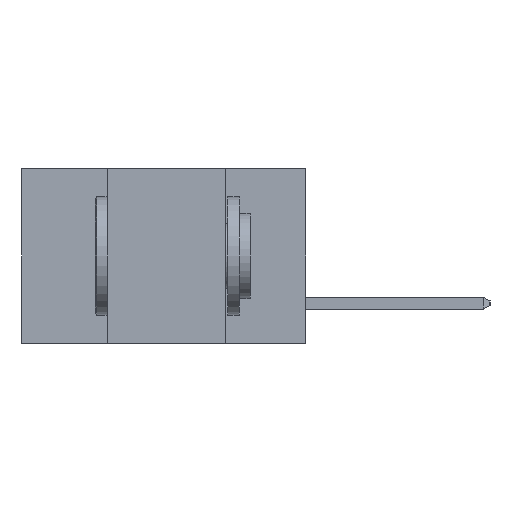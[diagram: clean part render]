
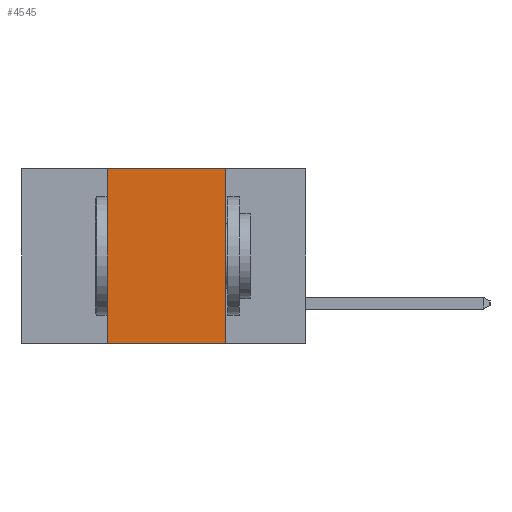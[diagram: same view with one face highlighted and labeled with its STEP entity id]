
A CAD part, left-side view. The second image highlights one B-rep face of the part: STEP entity #4545.
In plain terms, the highlighted planar face has unit normal (-1, 0, 0).
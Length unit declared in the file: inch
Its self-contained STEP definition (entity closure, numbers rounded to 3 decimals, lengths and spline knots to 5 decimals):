
#426 = LINE ( 'NONE', #20984, #14366 ) ;
#1055 = DIRECTION ( 'NONE',  ( 0., 0., 1. ) ) ;
#1083 = CARTESIAN_POINT ( 'NONE',  ( 0., 0.42, -0.37 ) ) ;
#1262 = EDGE_CURVE ( 'NONE', #13277, #11689, #426, .T. ) ;
#2244 = FACE_OUTER_BOUND ( 'NONE', #10930, .T. ) ;
#2871 = DIRECTION ( 'NONE',  ( 0., 0., -1. ) ) ;
#3153 = ORIENTED_EDGE ( 'NONE', *, *, #7551, .F. ) ;
#3324 = CARTESIAN_POINT ( 'NONE',  ( 0., 0.17, -0.37 ) ) ;
#3394 = LINE ( 'NONE', #14485, #21994 ) ;
#4510 = EDGE_CURVE ( 'NONE', #10075, #11689, #12654, .T. ) ;
#4545 = ADVANCED_FACE ( 'NONE', ( #2244 ), #21687, .F. ) ;
#5328 = ORIENTED_EDGE ( 'NONE', *, *, #4510, .F. ) ;
#5623 = CARTESIAN_POINT ( 'NONE',  ( 0., 0.17, 0. ) ) ;
#7551 = EDGE_CURVE ( 'NONE', #13277, #8636, #20561, .T. ) ;
#8636 = VERTEX_POINT ( 'NONE', #11726 ) ;
#8862 = ORIENTED_EDGE ( 'NONE', *, *, #17502, .F. ) ;
#10075 = VERTEX_POINT ( 'NONE', #5623 ) ;
#10930 = EDGE_LOOP ( 'NONE', ( #5328, #8862, #3153, #20760 ) ) ;
#11680 = VECTOR ( 'NONE', #1055, 39.37008 ) ;
#11689 = VERTEX_POINT ( 'NONE', #12304 ) ;
#11726 = CARTESIAN_POINT ( 'NONE',  ( 0., 0.42, 0. ) ) ;
#12304 = CARTESIAN_POINT ( 'NONE',  ( 0., 0.17, -0.37 ) ) ;
#12654 = LINE ( 'NONE', #3324, #16607 ) ;
#12837 = DIRECTION ( 'NONE',  ( 0., -1., 0. ) ) ;
#13277 = VERTEX_POINT ( 'NONE', #13948 ) ;
#13948 = CARTESIAN_POINT ( 'NONE',  ( 0., 0.42, -0.37 ) ) ;
#14366 = VECTOR ( 'NONE', #21563, 39.37008 ) ;
#14485 = CARTESIAN_POINT ( 'NONE',  ( 0., 0.6, 0. ) ) ;
#15072 = AXIS2_PLACEMENT_3D ( 'NONE', #21465, #21373, #21761 ) ;
#16607 = VECTOR ( 'NONE', #2871, 39.37008 ) ;
#17502 = EDGE_CURVE ( 'NONE', #8636, #10075, #3394, .T. ) ;
#20561 = LINE ( 'NONE', #1083, #11680 ) ;
#20760 = ORIENTED_EDGE ( 'NONE', *, *, #1262, .T. ) ;
#20984 = CARTESIAN_POINT ( 'NONE',  ( 0., 0.6, -0.37 ) ) ;
#21373 = DIRECTION ( 'NONE',  ( 1., 0., 0. ) ) ;
#21465 = CARTESIAN_POINT ( 'NONE',  ( 0., 0.6, 0. ) ) ;
#21563 = DIRECTION ( 'NONE',  ( 0., -1., 0. ) ) ;
#21687 = PLANE ( 'NONE',  #15072 ) ;
#21761 = DIRECTION ( 'NONE',  ( 0., 0., -1. ) ) ;
#21994 = VECTOR ( 'NONE', #12837, 39.37008 ) ;
